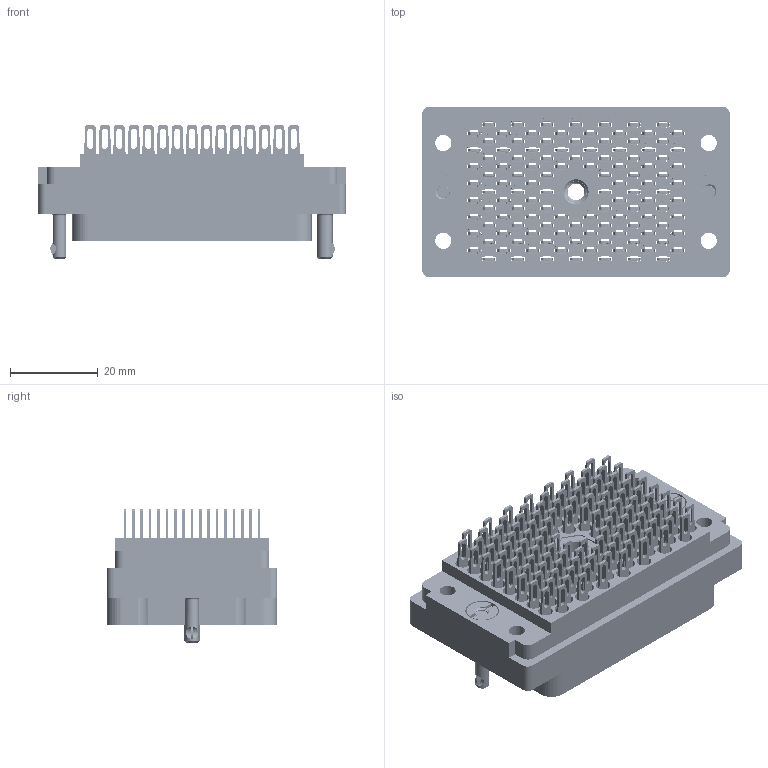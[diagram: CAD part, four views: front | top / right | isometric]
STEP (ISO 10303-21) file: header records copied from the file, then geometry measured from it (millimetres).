
FILE_DESCRIPTION (( 'STEP AP203' ), '1' );
FILE_NAME ('516-120-500-302.STEP', '2020-03-11T02:31:26', ( '' ), ( '' ), 'SwSTEP 2.0', 'SolidWorks 2016', '' );
FILE_SCHEMA (( 'CONFIG_CONTROL_DESIGN' ));
Length unit declared in the file: inch
Products named in the file (7): 516-222-090-102_091; 516-120-500-302; 516 Plug Insulator_120; 516-222-090-102_090; 516-252-091-102; 516-292-001_500 Contact; 516-252-095-100
Assembly tree (126 placements, depth 2):
  516-120-500-302
    516 Plug Insulator_120
    516-292-001_500 Contact  x120
    516-252-091-102  x2
    516-222-090-102_090
    516-252-095-100
    516-222-090-102_091
Bounding box: 69.85 x 38.73 x 30.33 mm (x, y, z)
Volume: 24593 mm3; surface area: 50142.6 mm2
Topology: 126 solids, 126 shells, 11723 faces, 34059 edges, 22607 vertices
Faces by surface type: plane 7014, cylinder 3903, bspline 756, cone 46, torus 4
Entity records: 100666 total; most frequent: CARTESIAN_POINT 23899, ORIENTED_EDGE 15602, DIRECTION 14884, EDGE_CURVE 7801, LINE 5724, VECTOR 5724, VERTEX_POINT 5181, AXIS2_PLACEMENT_3D 4580
